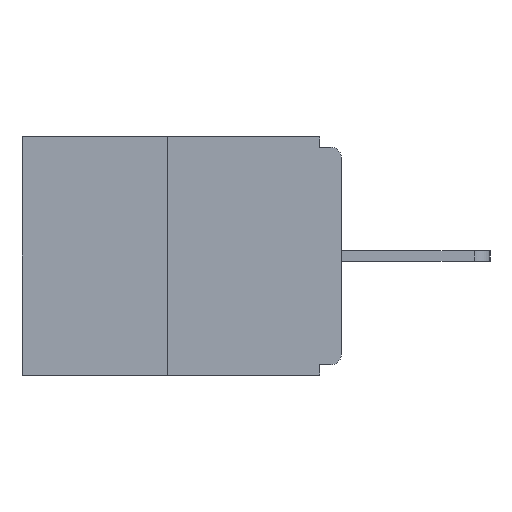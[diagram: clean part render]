
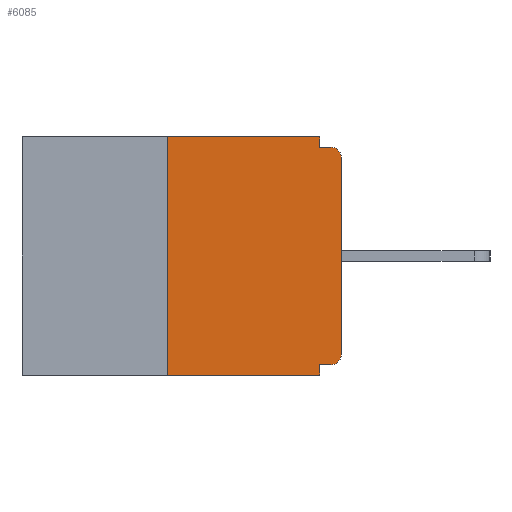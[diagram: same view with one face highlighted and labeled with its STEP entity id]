
A CAD part, left-side view. The second image highlights one B-rep face of the part: STEP entity #6085.
In plain terms, the highlighted planar face has unit normal (-1, 0, 0).
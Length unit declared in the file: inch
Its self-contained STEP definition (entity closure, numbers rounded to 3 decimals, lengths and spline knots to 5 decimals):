
#421 = ORIENTED_EDGE ( 'NONE', *, *, #10478, .T. ) ;
#671 = CARTESIAN_POINT ( 'NONE',  ( 0., 0.46, 0. ) ) ;
#850 = VECTOR ( 'NONE', #2403, 39.37008 ) ;
#903 = ORIENTED_EDGE ( 'NONE', *, *, #6598, .T. ) ;
#963 = DIRECTION ( 'NONE',  ( 0., 0., -1. ) ) ;
#1039 = CARTESIAN_POINT ( 'NONE',  ( 0., 0.25, -0.343 ) ) ;
#1189 = CARTESIAN_POINT ( 'NONE',  ( 0., 0.015, -0.03 ) ) ;
#2189 = CARTESIAN_POINT ( 'NONE',  ( 0., 0., -0.313 ) ) ;
#2264 = CARTESIAN_POINT ( 'NONE',  ( 0., 0.031, -0.015 ) ) ;
#2311 = EDGE_CURVE ( 'NONE', #13708, #5287, #10922, .T. ) ;
#2403 = DIRECTION ( 'NONE',  ( 0., 0., -1. ) ) ;
#2454 = ORIENTED_EDGE ( 'NONE', *, *, #10436, .F. ) ;
#2608 = CIRCLE ( 'NONE', #7111, 0.015 ) ;
#2614 = CARTESIAN_POINT ( 'NONE',  ( 0., 0.25, 0. ) ) ;
#2743 = CARTESIAN_POINT ( 'NONE',  ( 0., 0.25, 0. ) ) ;
#2852 = AXIS2_PLACEMENT_3D ( 'NONE', #671, #9272, #3238 ) ;
#2981 = DIRECTION ( 'NONE',  ( 0., 1., 0. ) ) ;
#3238 = DIRECTION ( 'NONE',  ( 0., 0., -1. ) ) ;
#3297 = CARTESIAN_POINT ( 'NONE',  ( 0., 0.015, -0.328 ) ) ;
#3336 = DIRECTION ( 'NONE',  ( -1., 0., 0. ) ) ;
#3391 = EDGE_CURVE ( 'NONE', #5152, #8263, #11643, .T. ) ;
#3659 = CARTESIAN_POINT ( 'NONE',  ( 0., 0., -0.015 ) ) ;
#3671 = LINE ( 'NONE', #8285, #4905 ) ;
#3741 = LINE ( 'NONE', #12342, #8607 ) ;
#4044 = DIRECTION ( 'NONE',  ( 0., -1., 0. ) ) ;
#4108 = EDGE_LOOP ( 'NONE', ( #4428, #2454, #13772, #14056, #5220, #5857, #421, #903, #14332, #11422 ) ) ;
#4428 = ORIENTED_EDGE ( 'NONE', *, *, #10133, .F. ) ;
#4736 = VERTEX_POINT ( 'NONE', #1039 ) ;
#4905 = VECTOR ( 'NONE', #4044, 39.37008 ) ;
#5008 = DIRECTION ( 'NONE',  ( 0., 0., 1. ) ) ;
#5152 = VERTEX_POINT ( 'NONE', #6724 ) ;
#5220 = ORIENTED_EDGE ( 'NONE', *, *, #13519, .F. ) ;
#5287 = VERTEX_POINT ( 'NONE', #2189 ) ;
#5362 = EDGE_CURVE ( 'NONE', #8263, #14124, #10914, .T. ) ;
#5762 = EDGE_CURVE ( 'NONE', #12141, #12420, #7095, .T. ) ;
#5857 = ORIENTED_EDGE ( 'NONE', *, *, #2311, .T. ) ;
#5993 = CARTESIAN_POINT ( 'NONE',  ( 0., 0.015, -0.015 ) ) ;
#6085 = ADVANCED_FACE ( 'NONE', ( #11665 ), #10338, .F. ) ;
#6166 = DIRECTION ( 'NONE',  ( 0., -1., 0. ) ) ;
#6242 = DIRECTION ( 'NONE',  ( -1., 0., 0. ) ) ;
#6506 = LINE ( 'NONE', #14946, #13074 ) ;
#6598 = EDGE_CURVE ( 'NONE', #8840, #14124, #2608, .T. ) ;
#6604 = VECTOR ( 'NONE', #7353, 39.37008 ) ;
#6685 = VECTOR ( 'NONE', #2981, 39.37008 ) ;
#6724 = CARTESIAN_POINT ( 'NONE',  ( 0., 0.031, 0. ) ) ;
#7095 = LINE ( 'NONE', #13017, #850 ) ;
#7111 = AXIS2_PLACEMENT_3D ( 'NONE', #1189, #6242, #13269 ) ;
#7116 = CARTESIAN_POINT ( 'NONE',  ( 0., 0.031, -0.343 ) ) ;
#7353 = DIRECTION ( 'NONE',  ( 0., 0., 1. ) ) ;
#7885 = CARTESIAN_POINT ( 'NONE',  ( 0., 0., -0.03 ) ) ;
#8263 = VERTEX_POINT ( 'NONE', #2264 ) ;
#8285 = CARTESIAN_POINT ( 'NONE',  ( 0., 0.46, -0.343 ) ) ;
#8444 = AXIS2_PLACEMENT_3D ( 'NONE', #12631, #3336, #13881 ) ;
#8607 = VECTOR ( 'NONE', #5008, 39.37008 ) ;
#8840 = VERTEX_POINT ( 'NONE', #7885 ) ;
#9125 = CARTESIAN_POINT ( 'NONE',  ( 0., 0.031, -0.328 ) ) ;
#9272 = DIRECTION ( 'NONE',  ( 1., 0., 0. ) ) ;
#10133 = EDGE_CURVE ( 'NONE', #13442, #5152, #6506, .T. ) ;
#10338 = PLANE ( 'NONE',  #2852 ) ;
#10436 = EDGE_CURVE ( 'NONE', #4736, #13442, #12180, .T. ) ;
#10478 = EDGE_CURVE ( 'NONE', #5287, #8840, #3741, .T. ) ;
#10914 = LINE ( 'NONE', #3659, #12042 ) ;
#10922 = CIRCLE ( 'NONE', #8444, 0.015 ) ;
#11422 = ORIENTED_EDGE ( 'NONE', *, *, #3391, .F. ) ;
#11643 = LINE ( 'NONE', #12976, #14503 ) ;
#11665 = FACE_OUTER_BOUND ( 'NONE', #4108, .T. ) ;
#12042 = VECTOR ( 'NONE', #6166, 39.37008 ) ;
#12043 = EDGE_CURVE ( 'NONE', #4736, #12420, #3671, .T. ) ;
#12141 = VERTEX_POINT ( 'NONE', #9125 ) ;
#12180 = LINE ( 'NONE', #2743, #6604 ) ;
#12342 = CARTESIAN_POINT ( 'NONE',  ( 0., 0., 0. ) ) ;
#12369 = LINE ( 'NONE', #12446, #6685 ) ;
#12420 = VERTEX_POINT ( 'NONE', #7116 ) ;
#12446 = CARTESIAN_POINT ( 'NONE',  ( 0., 0., -0.328 ) ) ;
#12631 = CARTESIAN_POINT ( 'NONE',  ( 0., 0.015, -0.313 ) ) ;
#12815 = DIRECTION ( 'NONE',  ( 0., -1., 0. ) ) ;
#12976 = CARTESIAN_POINT ( 'NONE',  ( 0., 0.031, 0. ) ) ;
#13017 = CARTESIAN_POINT ( 'NONE',  ( 0., 0.031, -0.343 ) ) ;
#13074 = VECTOR ( 'NONE', #12815, 39.37008 ) ;
#13269 = DIRECTION ( 'NONE',  ( 0., 0., -1. ) ) ;
#13442 = VERTEX_POINT ( 'NONE', #2614 ) ;
#13519 = EDGE_CURVE ( 'NONE', #13708, #12141, #12369, .T. ) ;
#13708 = VERTEX_POINT ( 'NONE', #3297 ) ;
#13772 = ORIENTED_EDGE ( 'NONE', *, *, #12043, .T. ) ;
#13881 = DIRECTION ( 'NONE',  ( 0., 0., -1. ) ) ;
#14056 = ORIENTED_EDGE ( 'NONE', *, *, #5762, .F. ) ;
#14124 = VERTEX_POINT ( 'NONE', #5993 ) ;
#14332 = ORIENTED_EDGE ( 'NONE', *, *, #5362, .F. ) ;
#14503 = VECTOR ( 'NONE', #963, 39.37008 ) ;
#14946 = CARTESIAN_POINT ( 'NONE',  ( 0., 0.46, 0. ) ) ;
